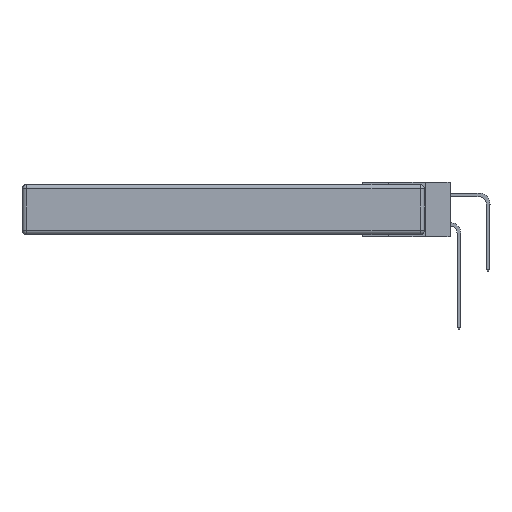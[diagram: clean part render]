
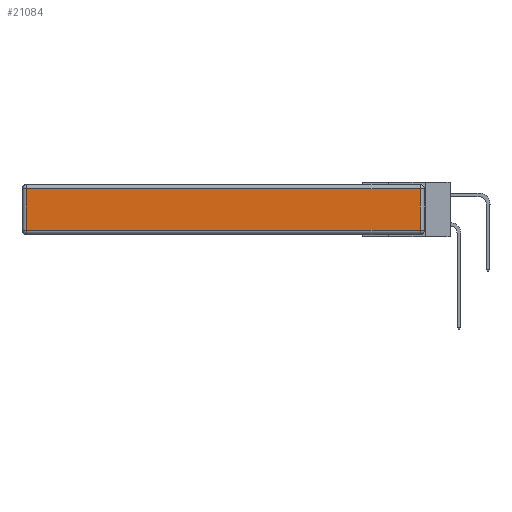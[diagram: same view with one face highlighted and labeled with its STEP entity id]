
A CAD part, left-side view. The second image highlights one B-rep face of the part: STEP entity #21084.
In plain terms, the highlighted planar face has unit normal (-1, 0, 0).
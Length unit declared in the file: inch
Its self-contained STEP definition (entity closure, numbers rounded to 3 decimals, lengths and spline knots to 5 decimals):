
#4 = VECTOR ( 'NONE', #3706, 39.37008 ) ;
#67 = PLANE ( 'NONE',  #9892 ) ;
#512 = DIRECTION ( 'NONE',  ( 0., 1., 0. ) ) ;
#1133 = DIRECTION ( 'NONE',  ( 0., -1., 0. ) ) ;
#1165 = EDGE_CURVE ( 'NONE', #9402, #17148, #22104, .T. ) ;
#2029 = LINE ( 'NONE', #14920, #5144 ) ;
#2060 = VERTEX_POINT ( 'NONE', #9789 ) ;
#3706 = DIRECTION ( 'NONE',  ( 0., 0., 1. ) ) ;
#5144 = VECTOR ( 'NONE', #25071, 39.37008 ) ;
#5200 = CARTESIAN_POINT ( 'NONE',  ( 0., 0., -0.343 ) ) ;
#5694 = EDGE_CURVE ( 'NONE', #17148, #2060, #2029, .T. ) ;
#9402 = VERTEX_POINT ( 'NONE', #27663 ) ;
#9789 = CARTESIAN_POINT ( 'NONE',  ( 0., 2.72, -0.313 ) ) ;
#9892 = AXIS2_PLACEMENT_3D ( 'NONE', #5200, #16088, #21036 ) ;
#11543 = ORIENTED_EDGE ( 'NONE', *, *, #1165, .T. ) ;
#12089 = VERTEX_POINT ( 'NONE', #21083 ) ;
#13414 = CARTESIAN_POINT ( 'NONE',  ( 0., 0., -0.313 ) ) ;
#14920 = CARTESIAN_POINT ( 'NONE',  ( 0., 2.72, -0.343 ) ) ;
#15294 = CARTESIAN_POINT ( 'NONE',  ( 0., 2.72, -0.03 ) ) ;
#16088 = DIRECTION ( 'NONE',  ( -1., 0., 0. ) ) ;
#17148 = VERTEX_POINT ( 'NONE', #15294 ) ;
#17603 = EDGE_CURVE ( 'NONE', #2060, #12089, #25034, .T. ) ;
#17827 = ORIENTED_EDGE ( 'NONE', *, *, #20257, .T. ) ;
#20257 = EDGE_CURVE ( 'NONE', #12089, #9402, #23710, .T. ) ;
#20843 = EDGE_LOOP ( 'NONE', ( #29832, #17827, #11543, #25962 ) ) ;
#21036 = DIRECTION ( 'NONE',  ( 0., 0., 1. ) ) ;
#21083 = CARTESIAN_POINT ( 'NONE',  ( 0., 0.03, -0.313 ) ) ;
#21084 = ADVANCED_FACE ( 'NONE', ( #29419 ), #67, .T. ) ;
#21325 = VECTOR ( 'NONE', #512, 39.37008 ) ;
#22104 = LINE ( 'NONE', #30167, #21325 ) ;
#23505 = VECTOR ( 'NONE', #1133, 39.37008 ) ;
#23710 = LINE ( 'NONE', #28937, #4 ) ;
#25034 = LINE ( 'NONE', #13414, #23505 ) ;
#25071 = DIRECTION ( 'NONE',  ( 0., 0., -1. ) ) ;
#25962 = ORIENTED_EDGE ( 'NONE', *, *, #5694, .T. ) ;
#27663 = CARTESIAN_POINT ( 'NONE',  ( 0., 0.03, -0.03 ) ) ;
#28937 = CARTESIAN_POINT ( 'NONE',  ( 0., 0.03, -0.343 ) ) ;
#29419 = FACE_OUTER_BOUND ( 'NONE', #20843, .T. ) ;
#29832 = ORIENTED_EDGE ( 'NONE', *, *, #17603, .T. ) ;
#30167 = CARTESIAN_POINT ( 'NONE',  ( 0., 2.75, -0.03 ) ) ;
